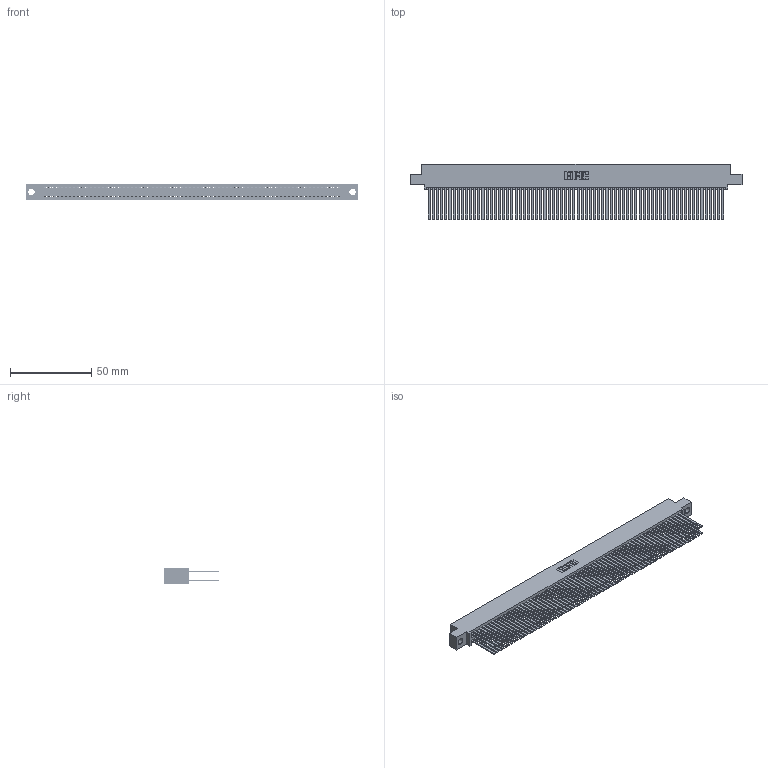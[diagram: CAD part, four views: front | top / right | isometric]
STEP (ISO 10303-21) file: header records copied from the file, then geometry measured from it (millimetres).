
FILE_DESCRIPTION (( 'STEP AP203' ), '1' );
FILE_NAME ('345-144-544-504.STEP', '2021-05-26T03:06:14', ( '' ), ( '' ), 'SwSTEP 2.0', 'SolidWorks 2020', '' );
FILE_SCHEMA (( 'CONFIG_CONTROL_DESIGN' ));
Length unit declared in the file: inch
Products named in the file (3): 345-144-544-504; 345-292-001_345-293-144; 345 Part_0.110 Offset - 0.156 Dia-TI
Assembly tree (145 placements, depth 2):
  345-144-544-504
    345 Part_0.110 Offset - 0.156 Dia-TI
    345-292-001_345-293-144  x144
Bounding box: 204.09 x 33.96 x 9.4 mm (x, y, z)
Volume: 21943.2 mm3; surface area: 38877.6 mm2
Topology: 145 solids, 145 shells, 6480 faces, 19253 edges, 12642 vertices
Faces by surface type: plane 4274, cylinder 2206
Entity records: 52821 total; most frequent: CARTESIAN_POINT 8830, ORIENTED_EDGE 8762, DIRECTION 7745, EDGE_CURVE 4381, VECTOR 3965, LINE 3965, VERTEX_POINT 2918, AXIS2_PLACEMENT_3D 1890
